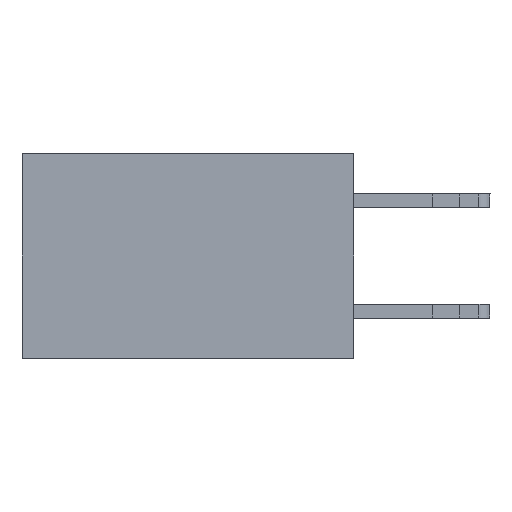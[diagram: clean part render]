
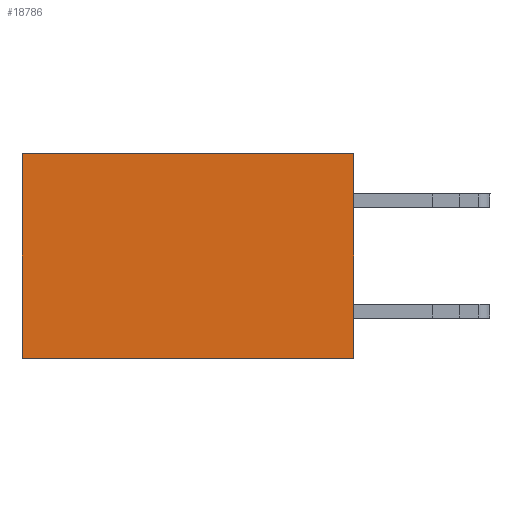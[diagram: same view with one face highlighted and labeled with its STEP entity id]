
A CAD part, left-side view. The second image highlights one B-rep face of the part: STEP entity #18786.
In plain terms, the highlighted planar face has unit normal (-1, 0, 0).
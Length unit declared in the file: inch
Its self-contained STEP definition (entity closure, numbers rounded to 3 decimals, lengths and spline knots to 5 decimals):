
#1140 = AXIS2_PLACEMENT_3D ( 'NONE', #8563, #22230, #6055 ) ;
#1275 = VERTEX_POINT ( 'NONE', #15097 ) ;
#1433 = EDGE_CURVE ( 'NONE', #28492, #13744, #12861, .T. ) ;
#3711 = DIRECTION ( 'NONE',  ( 0., 0., -1. ) ) ;
#4091 = LINE ( 'NONE', #25022, #7497 ) ;
#4821 = EDGE_CURVE ( 'NONE', #13744, #1275, #14990, .T. ) ;
#6055 = DIRECTION ( 'NONE',  ( 0., 0., -1. ) ) ;
#6370 = CARTESIAN_POINT ( 'NONE',  ( 0.2875, 0., -0.37 ) ) ;
#7497 = VECTOR ( 'NONE', #27616, 39.37008 ) ;
#8077 = CARTESIAN_POINT ( 'NONE',  ( 0.2875, 0., 0. ) ) ;
#8563 = CARTESIAN_POINT ( 'NONE',  ( 0.2875, 0., 0. ) ) ;
#8922 = VECTOR ( 'NONE', #3711, 39.37008 ) ;
#10127 = ORIENTED_EDGE ( 'NONE', *, *, #1433, .F. ) ;
#12441 = VECTOR ( 'NONE', #20042, 39.37008 ) ;
#12499 = EDGE_LOOP ( 'NONE', ( #21446, #19348, #10127, #29012 ) ) ;
#12861 = LINE ( 'NONE', #8077, #31964 ) ;
#13744 = VERTEX_POINT ( 'NONE', #26079 ) ;
#14990 = LINE ( 'NONE', #6370, #12441 ) ;
#15097 = CARTESIAN_POINT ( 'NONE',  ( 0.2875, 0.6, -0.37 ) ) ;
#15136 = CARTESIAN_POINT ( 'NONE',  ( 0.2875, 0.6, 0. ) ) ;
#18786 = ADVANCED_FACE ( 'NONE', ( #27782 ), #19384, .F. ) ;
#19348 = ORIENTED_EDGE ( 'NONE', *, *, #4821, .F. ) ;
#19384 = PLANE ( 'NONE',  #1140 ) ;
#20042 = DIRECTION ( 'NONE',  ( 0., 1., 0. ) ) ;
#21446 = ORIENTED_EDGE ( 'NONE', *, *, #29897, .T. ) ;
#22230 = DIRECTION ( 'NONE',  ( 1., 0., 0. ) ) ;
#24074 = CARTESIAN_POINT ( 'NONE',  ( 0.2875, 0.6, 0. ) ) ;
#25022 = CARTESIAN_POINT ( 'NONE',  ( 0.2875, 0., 0. ) ) ;
#25875 = DIRECTION ( 'NONE',  ( 0., 0., -1. ) ) ;
#26079 = CARTESIAN_POINT ( 'NONE',  ( 0.2875, 0., -0.37 ) ) ;
#26944 = EDGE_CURVE ( 'NONE', #28492, #30866, #4091, .T. ) ;
#27616 = DIRECTION ( 'NONE',  ( 0., 1., 0. ) ) ;
#27782 = FACE_OUTER_BOUND ( 'NONE', #12499, .T. ) ;
#28492 = VERTEX_POINT ( 'NONE', #28755 ) ;
#28755 = CARTESIAN_POINT ( 'NONE',  ( 0.2875, 0., 0. ) ) ;
#29012 = ORIENTED_EDGE ( 'NONE', *, *, #26944, .T. ) ;
#29897 = EDGE_CURVE ( 'NONE', #30866, #1275, #31019, .T. ) ;
#30866 = VERTEX_POINT ( 'NONE', #24074 ) ;
#31019 = LINE ( 'NONE', #15136, #8922 ) ;
#31964 = VECTOR ( 'NONE', #25875, 39.37008 ) ;
